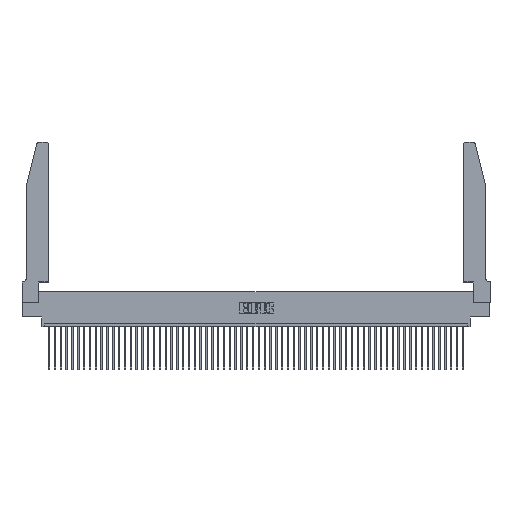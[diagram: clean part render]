
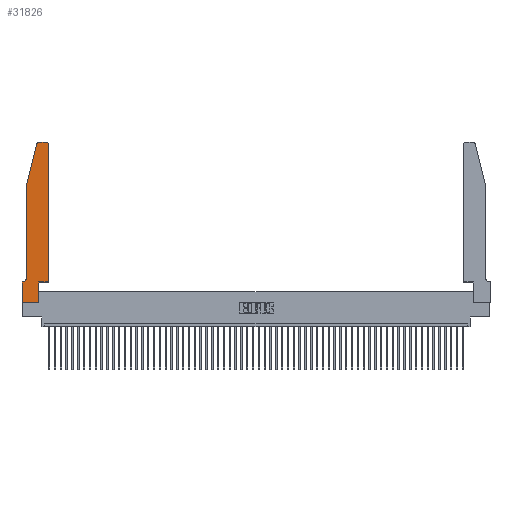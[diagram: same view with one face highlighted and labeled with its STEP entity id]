
A CAD part, top view. The second image highlights one B-rep face of the part: STEP entity #31826.
In plain terms, the highlighted planar face has unit normal (0, 0, 1).
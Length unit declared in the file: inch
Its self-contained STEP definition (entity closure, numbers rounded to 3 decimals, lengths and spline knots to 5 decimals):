
#741 = CARTESIAN_POINT ( 'NONE',  ( 0.0755, 0.42, 0.37 ) ) ;
#1205 = ORIENTED_EDGE ( 'NONE', *, *, #21750, .T. ) ;
#1388 = AXIS2_PLACEMENT_3D ( 'NONE', #21593, #30597, #26575 ) ;
#1544 = CARTESIAN_POINT ( 'NONE',  ( 0.4505, 2.72, 0.37 ) ) ;
#2891 = LINE ( 'NONE', #49665, #35425 ) ;
#3961 = EDGE_CURVE ( 'NONE', #44894, #23102, #34201, .T. ) ;
#4106 = ORIENTED_EDGE ( 'NONE', *, *, #24300, .T. ) ;
#4796 = ORIENTED_EDGE ( 'NONE', *, *, #13402, .T. ) ;
#5346 = DIRECTION ( 'NONE',  ( -1., 0., 0. ) ) ;
#6860 = VERTEX_POINT ( 'NONE', #24090 ) ;
#7654 = DIRECTION ( 'NONE',  ( 1., 0., 0. ) ) ;
#7985 = AXIS2_PLACEMENT_3D ( 'NONE', #16553, #24327, #24513 ) ;
#8708 = VECTOR ( 'NONE', #27990, 39.37008 ) ;
#9577 = ORIENTED_EDGE ( 'NONE', *, *, #10473, .T. ) ;
#10276 = ORIENTED_EDGE ( 'NONE', *, *, #32701, .T. ) ;
#10473 = EDGE_CURVE ( 'NONE', #45378, #6860, #48258, .T. ) ;
#10532 = VECTOR ( 'NONE', #31385, 39.37008 ) ;
#10919 = DIRECTION ( 'NONE',  ( -1., 0., 0. ) ) ;
#11152 = EDGE_CURVE ( 'NONE', #22891, #17408, #51889, .T. ) ;
#11676 = CIRCLE ( 'NONE', #28507, 0.03 ) ;
#13402 = EDGE_CURVE ( 'NONE', #33507, #33196, #40435, .T. ) ;
#13674 = LINE ( 'NONE', #19721, #40993 ) ;
#13755 = CARTESIAN_POINT ( 'NONE',  ( 0., 0., 0.37 ) ) ;
#14255 = CARTESIAN_POINT ( 'NONE',  ( 0.2865, 0.35, 0.37 ) ) ;
#14603 = CARTESIAN_POINT ( 'NONE',  ( 0.0055, 0.35, 0.37 ) ) ;
#16553 = CARTESIAN_POINT ( 'NONE',  ( 0.284, 2.72, 0.37 ) ) ;
#17162 = DIRECTION ( 'NONE',  ( 1., 0., 0. ) ) ;
#17408 = VERTEX_POINT ( 'NONE', #19147 ) ;
#17474 = CARTESIAN_POINT ( 'NONE',  ( 0.4205, 2.75, 0.37 ) ) ;
#17488 = CARTESIAN_POINT ( 'NONE',  ( 0.4205, 2.72, 0.37 ) ) ;
#17923 = EDGE_CURVE ( 'NONE', #31261, #22891, #13674, .T. ) ;
#19147 = CARTESIAN_POINT ( 'NONE',  ( 0.4505, 0.35, 0.37 ) ) ;
#19721 = CARTESIAN_POINT ( 'NONE',  ( 0.2865, 0.35, 0.37 ) ) ;
#20065 = LINE ( 'NONE', #28247, #8708 ) ;
#20810 = VECTOR ( 'NONE', #7654, 39.37008 ) ;
#21593 = CARTESIAN_POINT ( 'NONE',  ( 0., 0.35, 0.37 ) ) ;
#21750 = EDGE_CURVE ( 'NONE', #6860, #49508, #20065, .T. ) ;
#22180 = VECTOR ( 'NONE', #23316, 39.37008 ) ;
#22891 = VERTEX_POINT ( 'NONE', #14255 ) ;
#23067 = ORIENTED_EDGE ( 'NONE', *, *, #17923, .T. ) ;
#23102 = VERTEX_POINT ( 'NONE', #47802 ) ;
#23316 = DIRECTION ( 'NONE',  ( 0., -1., 0. ) ) ;
#23369 = FACE_OUTER_BOUND ( 'NONE', #31871, .T. ) ;
#23548 = LINE ( 'NONE', #47959, #22180 ) ;
#24090 = CARTESIAN_POINT ( 'NONE',  ( 0., 0.35, 0.37 ) ) ;
#24201 = CARTESIAN_POINT ( 'NONE',  ( 0.4505, 0.35, 0.37 ) ) ;
#24300 = EDGE_CURVE ( 'NONE', #52533, #45378, #40040, .T. ) ;
#24327 = DIRECTION ( 'NONE',  ( 0., 0., 1. ) ) ;
#24513 = DIRECTION ( 'NONE',  ( 1., 0., 0. ) ) ;
#25888 = DIRECTION ( 'NONE',  ( 0., 0., 1. ) ) ;
#26572 = DIRECTION ( 'NONE',  ( 0., 0., -1. ) ) ;
#26575 = DIRECTION ( 'NONE',  ( 1., 0., 0. ) ) ;
#27463 = VERTEX_POINT ( 'NONE', #1544 ) ;
#27609 = ORIENTED_EDGE ( 'NONE', *, *, #53439, .T. ) ;
#27990 = DIRECTION ( 'NONE',  ( 0., -1., 0. ) ) ;
#28247 = CARTESIAN_POINT ( 'NONE',  ( 0., 0., 0.37 ) ) ;
#28507 = AXIS2_PLACEMENT_3D ( 'NONE', #17488, #25888, #17162 ) ;
#28534 = EDGE_CURVE ( 'NONE', #27463, #33507, #11676, .T. ) ;
#29539 = CARTESIAN_POINT ( 'NONE',  ( 0., 0., 0.37 ) ) ;
#29764 = CARTESIAN_POINT ( 'NONE',  ( 0.0055, 0.42, 0.37 ) ) ;
#30597 = DIRECTION ( 'NONE',  ( 0., 0., 1. ) ) ;
#31261 = VERTEX_POINT ( 'NONE', #43508 ) ;
#31385 = DIRECTION ( 'NONE',  ( -1., 0., 0. ) ) ;
#31826 = ADVANCED_FACE ( 'NONE', ( #23369 ), #51437, .T. ) ;
#31871 = EDGE_LOOP ( 'NONE', ( #4796, #10276, #36612, #32687, #4106, #9577, #1205, #43407, #23067, #51453, #27609, #35511 ) ) ;
#31939 = CARTESIAN_POINT ( 'NONE',  ( 0.2605, 2.75, 0.37 ) ) ;
#32382 = CARTESIAN_POINT ( 'NONE',  ( 0.25487, 2.72718, 0.37 ) ) ;
#32687 = ORIENTED_EDGE ( 'NONE', *, *, #46003, .T. ) ;
#32701 = EDGE_CURVE ( 'NONE', #33196, #44894, #49141, .T. ) ;
#33196 = VERTEX_POINT ( 'NONE', #48299 ) ;
#33507 = VERTEX_POINT ( 'NONE', #17474 ) ;
#34201 = LINE ( 'NONE', #48647, #37581 ) ;
#35425 = VECTOR ( 'NONE', #41858, 39.37008 ) ;
#35511 = ORIENTED_EDGE ( 'NONE', *, *, #28534, .T. ) ;
#36250 = DIRECTION ( 'NONE',  ( -0.239, -0.971, 0. ) ) ;
#36574 = LINE ( 'NONE', #13755, #46535 ) ;
#36612 = ORIENTED_EDGE ( 'NONE', *, *, #3961, .T. ) ;
#37581 = VECTOR ( 'NONE', #36250, 39.37008 ) ;
#40040 = CIRCLE ( 'NONE', #54666, 0.07 ) ;
#40435 = LINE ( 'NONE', #31939, #10532 ) ;
#40993 = VECTOR ( 'NONE', #50316, 39.37008 ) ;
#41858 = DIRECTION ( 'NONE',  ( 0., 1., 0. ) ) ;
#43407 = ORIENTED_EDGE ( 'NONE', *, *, #48834, .T. ) ;
#43498 = DIRECTION ( 'NONE',  ( 1., 0., 0. ) ) ;
#43508 = CARTESIAN_POINT ( 'NONE',  ( 0.2865, 0., 0.37 ) ) ;
#44265 = VECTOR ( 'NONE', #10919, 39.37008 ) ;
#44706 = CARTESIAN_POINT ( 'NONE',  ( 0.0755, 0.35, 0.37 ) ) ;
#44894 = VERTEX_POINT ( 'NONE', #32382 ) ;
#45378 = VERTEX_POINT ( 'NONE', #14603 ) ;
#46003 = EDGE_CURVE ( 'NONE', #23102, #52533, #23548, .T. ) ;
#46535 = VECTOR ( 'NONE', #43498, 39.37008 ) ;
#47802 = CARTESIAN_POINT ( 'NONE',  ( 0.0755, 2., 0.37 ) ) ;
#47959 = CARTESIAN_POINT ( 'NONE',  ( 0.0755, 2., 0.37 ) ) ;
#48258 = LINE ( 'NONE', #44706, #44265 ) ;
#48299 = CARTESIAN_POINT ( 'NONE',  ( 0.284, 2.75, 0.37 ) ) ;
#48647 = CARTESIAN_POINT ( 'NONE',  ( 0.0755, 2., 0.37 ) ) ;
#48834 = EDGE_CURVE ( 'NONE', #49508, #31261, #36574, .T. ) ;
#49141 = CIRCLE ( 'NONE', #7985, 0.03 ) ;
#49508 = VERTEX_POINT ( 'NONE', #29539 ) ;
#49665 = CARTESIAN_POINT ( 'NONE',  ( 0.4505, 0.35, 0.37 ) ) ;
#50316 = DIRECTION ( 'NONE',  ( 0., 1., 0. ) ) ;
#51437 = PLANE ( 'NONE',  #1388 ) ;
#51453 = ORIENTED_EDGE ( 'NONE', *, *, #11152, .T. ) ;
#51889 = LINE ( 'NONE', #24201, #20810 ) ;
#52533 = VERTEX_POINT ( 'NONE', #741 ) ;
#53439 = EDGE_CURVE ( 'NONE', #17408, #27463, #2891, .T. ) ;
#54666 = AXIS2_PLACEMENT_3D ( 'NONE', #29764, #26572, #5346 ) ;
